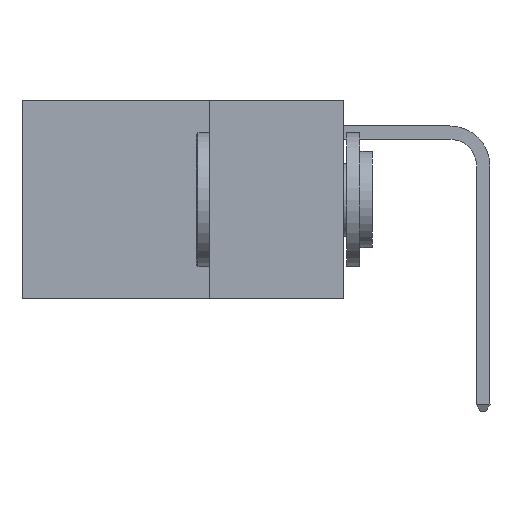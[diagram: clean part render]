
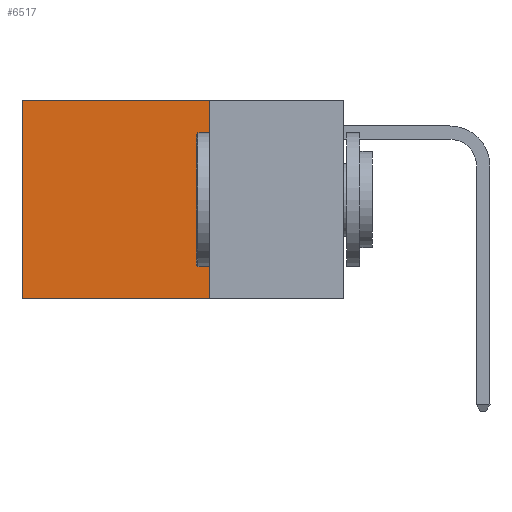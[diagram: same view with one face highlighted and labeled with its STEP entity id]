
A CAD part, left-side view. The second image highlights one B-rep face of the part: STEP entity #6517.
In plain terms, the highlighted planar face has unit normal (-1, 0, 0).
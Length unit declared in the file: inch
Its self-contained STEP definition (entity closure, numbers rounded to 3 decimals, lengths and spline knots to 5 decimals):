
#424 = VERTEX_POINT ( 'NONE', #12631 ) ;
#1157 = ORIENTED_EDGE ( 'NONE', *, *, #7090, .T. ) ;
#2126 = VECTOR ( 'NONE', #14697, 39.37008 ) ;
#2475 = CARTESIAN_POINT ( 'NONE',  ( 0.2625, 0.25, 0. ) ) ;
#4256 = DIRECTION ( 'NONE',  ( 1., 0., 0. ) ) ;
#4300 = LINE ( 'NONE', #2475, #2126 ) ;
#5101 = VERTEX_POINT ( 'NONE', #6075 ) ;
#5494 = ORIENTED_EDGE ( 'NONE', *, *, #20627, .T. ) ;
#6075 = CARTESIAN_POINT ( 'NONE',  ( 0.2625, 0.6, -0.37 ) ) ;
#6517 = ADVANCED_FACE ( 'NONE', ( #21055 ), #14253, .F. ) ;
#7090 = EDGE_CURVE ( 'NONE', #19127, #424, #17720, .T. ) ;
#7463 = DIRECTION ( 'NONE',  ( 0., 0., -1. ) ) ;
#7719 = VERTEX_POINT ( 'NONE', #12682 ) ;
#8596 = VECTOR ( 'NONE', #7463, 39.37008 ) ;
#9038 = VECTOR ( 'NONE', #19052, 39.37008 ) ;
#10228 = LINE ( 'NONE', #16905, #21603 ) ;
#12342 = ORIENTED_EDGE ( 'NONE', *, *, #21498, .F. ) ;
#12631 = CARTESIAN_POINT ( 'NONE',  ( 0.2625, 0.6, 0. ) ) ;
#12682 = CARTESIAN_POINT ( 'NONE',  ( 0.2625, 0.25, -0.37 ) ) ;
#14253 = PLANE ( 'NONE',  #14426 ) ;
#14426 = AXIS2_PLACEMENT_3D ( 'NONE', #19774, #4256, #21581 ) ;
#14697 = DIRECTION ( 'NONE',  ( 0., 0., -1. ) ) ;
#15631 = LINE ( 'NONE', #19467, #8596 ) ;
#16001 = EDGE_LOOP ( 'NONE', ( #5494, #18263, #12342, #1157 ) ) ;
#16008 = CARTESIAN_POINT ( 'NONE',  ( 0.2625, 0.25, 0. ) ) ;
#16905 = CARTESIAN_POINT ( 'NONE',  ( 0.2625, 0.25, -0.37 ) ) ;
#17132 = DIRECTION ( 'NONE',  ( 0., 1., 0. ) ) ;
#17245 = EDGE_CURVE ( 'NONE', #7719, #5101, #10228, .T. ) ;
#17720 = LINE ( 'NONE', #16008, #9038 ) ;
#18263 = ORIENTED_EDGE ( 'NONE', *, *, #17245, .F. ) ;
#19052 = DIRECTION ( 'NONE',  ( 0., 1., 0. ) ) ;
#19127 = VERTEX_POINT ( 'NONE', #19346 ) ;
#19346 = CARTESIAN_POINT ( 'NONE',  ( 0.2625, 0.25, 0. ) ) ;
#19467 = CARTESIAN_POINT ( 'NONE',  ( 0.2625, 0.6, 0. ) ) ;
#19774 = CARTESIAN_POINT ( 'NONE',  ( 0.2625, 0.25, 0. ) ) ;
#20627 = EDGE_CURVE ( 'NONE', #424, #5101, #15631, .T. ) ;
#21055 = FACE_OUTER_BOUND ( 'NONE', #16001, .T. ) ;
#21498 = EDGE_CURVE ( 'NONE', #19127, #7719, #4300, .T. ) ;
#21581 = DIRECTION ( 'NONE',  ( 0., 0., -1. ) ) ;
#21603 = VECTOR ( 'NONE', #17132, 39.37008 ) ;
